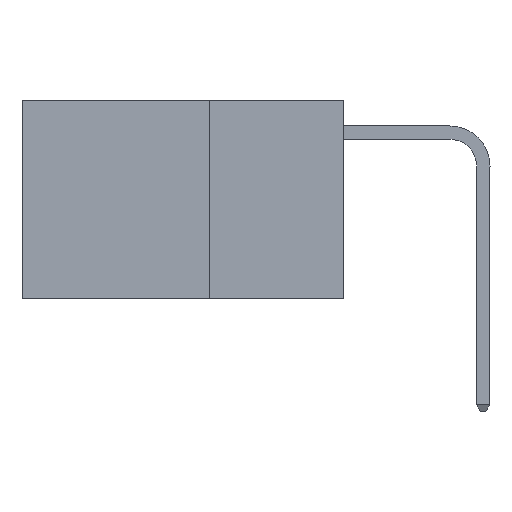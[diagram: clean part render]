
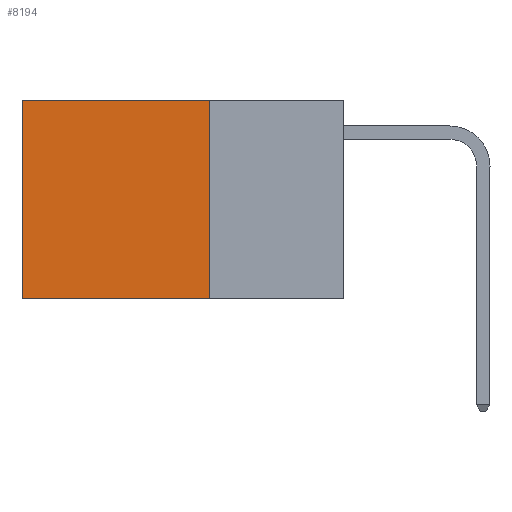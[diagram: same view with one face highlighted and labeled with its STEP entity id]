
A CAD part, left-side view. The second image highlights one B-rep face of the part: STEP entity #8194.
In plain terms, the highlighted planar face has unit normal (-1, 0, 0).
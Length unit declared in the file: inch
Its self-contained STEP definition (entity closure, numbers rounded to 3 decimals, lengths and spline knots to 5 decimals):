
#142 = DIRECTION ( 'NONE',  ( 0., 0., -1. ) ) ;
#311 = DIRECTION ( 'NONE',  ( 0., 1., 0. ) ) ;
#513 = CARTESIAN_POINT ( 'NONE',  ( 0.2625, 0.25, 0. ) ) ;
#1146 = VECTOR ( 'NONE', #311, 39.37008 ) ;
#1870 = VERTEX_POINT ( 'NONE', #12574 ) ;
#1927 = EDGE_CURVE ( 'NONE', #14610, #1870, #5973, .T. ) ;
#3197 = EDGE_CURVE ( 'NONE', #8385, #14610, #12677, .T. ) ;
#3371 = VERTEX_POINT ( 'NONE', #12717 ) ;
#4733 = LINE ( 'NONE', #5112, #1146 ) ;
#4985 = CARTESIAN_POINT ( 'NONE',  ( 0.2625, 0.6, 0. ) ) ;
#5071 = DIRECTION ( 'NONE',  ( 0., 0., -1. ) ) ;
#5112 = CARTESIAN_POINT ( 'NONE',  ( 0.2625, 0.25, -0.37 ) ) ;
#5156 = EDGE_LOOP ( 'NONE', ( #8932, #14646, #7489, #11059 ) ) ;
#5633 = EDGE_CURVE ( 'NONE', #3371, #1870, #4733, .T. ) ;
#5973 = LINE ( 'NONE', #7115, #11974 ) ;
#6153 = CARTESIAN_POINT ( 'NONE',  ( 0.2625, 0.25, 0. ) ) ;
#6424 = CARTESIAN_POINT ( 'NONE',  ( 0.2625, 0.25, 0. ) ) ;
#6664 = VECTOR ( 'NONE', #13572, 39.37008 ) ;
#7093 = AXIS2_PLACEMENT_3D ( 'NONE', #6153, #7320, #142 ) ;
#7115 = CARTESIAN_POINT ( 'NONE',  ( 0.2625, 0.6, 0. ) ) ;
#7320 = DIRECTION ( 'NONE',  ( 1., 0., 0. ) ) ;
#7489 = ORIENTED_EDGE ( 'NONE', *, *, #14514, .F. ) ;
#7747 = VECTOR ( 'NONE', #15406, 39.37008 ) ;
#8138 = LINE ( 'NONE', #10761, #7747 ) ;
#8194 = ADVANCED_FACE ( 'NONE', ( #9337 ), #14477, .F. ) ;
#8385 = VERTEX_POINT ( 'NONE', #513 ) ;
#8932 = ORIENTED_EDGE ( 'NONE', *, *, #1927, .T. ) ;
#9337 = FACE_OUTER_BOUND ( 'NONE', #5156, .T. ) ;
#10761 = CARTESIAN_POINT ( 'NONE',  ( 0.2625, 0.25, 0. ) ) ;
#11059 = ORIENTED_EDGE ( 'NONE', *, *, #3197, .T. ) ;
#11974 = VECTOR ( 'NONE', #5071, 39.37008 ) ;
#12574 = CARTESIAN_POINT ( 'NONE',  ( 0.2625, 0.6, -0.37 ) ) ;
#12677 = LINE ( 'NONE', #6424, #6664 ) ;
#12717 = CARTESIAN_POINT ( 'NONE',  ( 0.2625, 0.25, -0.37 ) ) ;
#13572 = DIRECTION ( 'NONE',  ( 0., 1., 0. ) ) ;
#14477 = PLANE ( 'NONE',  #7093 ) ;
#14514 = EDGE_CURVE ( 'NONE', #8385, #3371, #8138, .T. ) ;
#14610 = VERTEX_POINT ( 'NONE', #4985 ) ;
#14646 = ORIENTED_EDGE ( 'NONE', *, *, #5633, .F. ) ;
#15406 = DIRECTION ( 'NONE',  ( 0., 0., -1. ) ) ;
